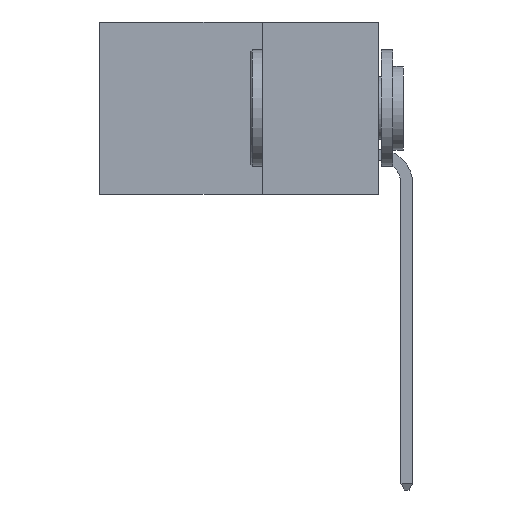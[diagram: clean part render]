
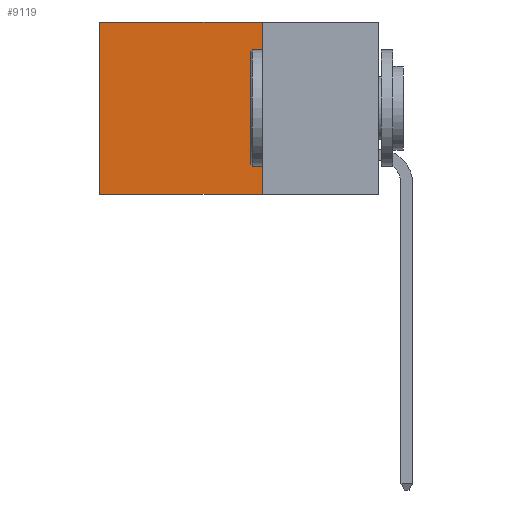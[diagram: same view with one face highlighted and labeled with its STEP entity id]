
A CAD part, left-side view. The second image highlights one B-rep face of the part: STEP entity #9119.
In plain terms, the highlighted planar face has unit normal (-1, 0, 0).
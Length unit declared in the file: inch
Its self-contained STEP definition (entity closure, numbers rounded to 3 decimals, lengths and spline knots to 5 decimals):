
#148 = VERTEX_POINT ( 'NONE', #12261 ) ;
#229 = CARTESIAN_POINT ( 'NONE',  ( 0.2615, 0.6, -0.37 ) ) ;
#511 = EDGE_LOOP ( 'NONE', ( #6043, #4964, #9493, #11230 ) ) ;
#654 = EDGE_CURVE ( 'NONE', #148, #11041, #12382, .T. ) ;
#2103 = LINE ( 'NONE', #12890, #13963 ) ;
#2242 = CARTESIAN_POINT ( 'NONE',  ( 0.2615, 0.25, -0.37 ) ) ;
#3146 = DIRECTION ( 'NONE',  ( 0., 0., -1. ) ) ;
#3617 = DIRECTION ( 'NONE',  ( 0., 1., 0. ) ) ;
#4306 = AXIS2_PLACEMENT_3D ( 'NONE', #4782, #9564, #13942 ) ;
#4527 = VERTEX_POINT ( 'NONE', #2242 ) ;
#4782 = CARTESIAN_POINT ( 'NONE',  ( 0.2615, 0.25, -0.37 ) ) ;
#4868 = VERTEX_POINT ( 'NONE', #229 ) ;
#4900 = LINE ( 'NONE', #5539, #12412 ) ;
#4964 = ORIENTED_EDGE ( 'NONE', *, *, #14586, .F. ) ;
#5539 = CARTESIAN_POINT ( 'NONE',  ( 0.2615, 0.25, -0.37 ) ) ;
#5769 = VECTOR ( 'NONE', #7095, 39.37008 ) ;
#6043 = ORIENTED_EDGE ( 'NONE', *, *, #10693, .T. ) ;
#7095 = DIRECTION ( 'NONE',  ( 0., 1., 0. ) ) ;
#7142 = CARTESIAN_POINT ( 'NONE',  ( 0.2615, 0.6, -0.37 ) ) ;
#7176 = PLANE ( 'NONE',  #4306 ) ;
#7756 = LINE ( 'NONE', #7142, #13883 ) ;
#8331 = EDGE_CURVE ( 'NONE', #148, #4527, #4900, .T. ) ;
#9119 = ADVANCED_FACE ( 'NONE', ( #11437 ), #7176, .F. ) ;
#9493 = ORIENTED_EDGE ( 'NONE', *, *, #8331, .F. ) ;
#9564 = DIRECTION ( 'NONE',  ( 1., 0., 0. ) ) ;
#10693 = EDGE_CURVE ( 'NONE', #11041, #4868, #7756, .T. ) ;
#11041 = VERTEX_POINT ( 'NONE', #12575 ) ;
#11230 = ORIENTED_EDGE ( 'NONE', *, *, #654, .T. ) ;
#11437 = FACE_OUTER_BOUND ( 'NONE', #511, .T. ) ;
#12261 = CARTESIAN_POINT ( 'NONE',  ( 0.2615, 0.25, 0. ) ) ;
#12382 = LINE ( 'NONE', #12699, #5769 ) ;
#12412 = VECTOR ( 'NONE', #3146, 39.37008 ) ;
#12575 = CARTESIAN_POINT ( 'NONE',  ( 0.2615, 0.6, 0. ) ) ;
#12699 = CARTESIAN_POINT ( 'NONE',  ( 0.2615, 0.25, 0. ) ) ;
#12890 = CARTESIAN_POINT ( 'NONE',  ( 0.2615, 0.25, -0.37 ) ) ;
#13883 = VECTOR ( 'NONE', #14117, 39.37008 ) ;
#13942 = DIRECTION ( 'NONE',  ( 0., 0., -1. ) ) ;
#13963 = VECTOR ( 'NONE', #3617, 39.37008 ) ;
#14117 = DIRECTION ( 'NONE',  ( 0., 0., -1. ) ) ;
#14586 = EDGE_CURVE ( 'NONE', #4527, #4868, #2103, .T. ) ;
